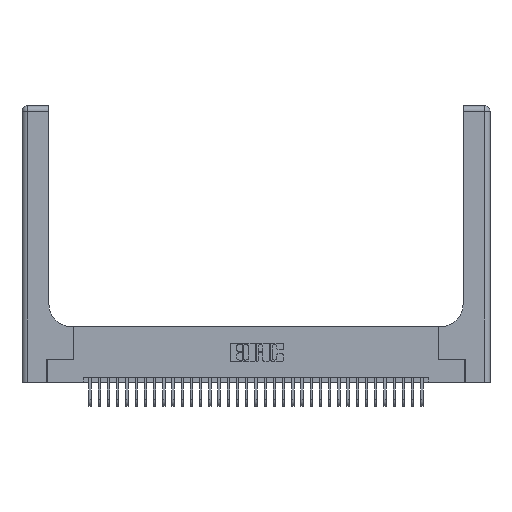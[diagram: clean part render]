
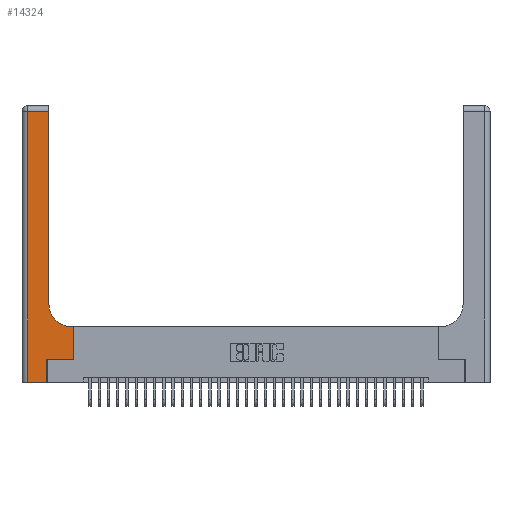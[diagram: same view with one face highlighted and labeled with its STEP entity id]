
A CAD part, top view. The second image highlights one B-rep face of the part: STEP entity #14324.
In plain terms, the highlighted planar face has unit normal (0, 0, 1).
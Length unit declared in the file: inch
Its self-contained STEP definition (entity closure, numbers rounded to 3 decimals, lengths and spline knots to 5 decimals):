
#932 = DIRECTION ( 'NONE',  ( 1., 0., 0. ) ) ;
#1067 = ORIENTED_EDGE ( 'NONE', *, *, #11201, .T. ) ;
#1811 = VECTOR ( 'NONE', #33774, 39.37008 ) ;
#1850 = CARTESIAN_POINT ( 'NONE',  ( 0., 0., 0.37 ) ) ;
#2205 = EDGE_CURVE ( 'NONE', #10153, #10173, #7530, .T. ) ;
#2216 = VECTOR ( 'NONE', #6789, 39.37008 ) ;
#2232 = ORIENTED_EDGE ( 'NONE', *, *, #28608, .T. ) ;
#2854 = VECTOR ( 'NONE', #29678, 39.37008 ) ;
#2979 = AXIS2_PLACEMENT_3D ( 'NONE', #20899, #5239, #23478 ) ;
#3751 = VECTOR ( 'NONE', #20194, 39.37008 ) ;
#5239 = DIRECTION ( 'NONE',  ( 0., 0., -1. ) ) ;
#5244 = EDGE_LOOP ( 'NONE', ( #20873, #32970, #9070, #2232, #15638, #33032, #24427, #32027, #1067 ) ) ;
#6436 = VERTEX_POINT ( 'NONE', #19688 ) ;
#6688 = CARTESIAN_POINT ( 'NONE',  ( 0.5585, 0.25, 0.37 ) ) ;
#6713 = EDGE_CURVE ( 'NONE', #10173, #20975, #14974, .T. ) ;
#6789 = DIRECTION ( 'NONE',  ( 0., 1., 0. ) ) ;
#6924 = DIRECTION ( 'NONE',  ( -1., 0., 0. ) ) ;
#6925 = EDGE_CURVE ( 'NONE', #18355, #10153, #29139, .T. ) ;
#7143 = CARTESIAN_POINT ( 'NONE',  ( 0.269, 0., 0.37 ) ) ;
#7530 = LINE ( 'NONE', #20809, #27480 ) ;
#7787 = CARTESIAN_POINT ( 'NONE',  ( 0.5585, 0.6, 0.37 ) ) ;
#8911 = CARTESIAN_POINT ( 'NONE',  ( 0.2915, 3., 0.37 ) ) ;
#8939 = CARTESIAN_POINT ( 'NONE',  ( 0.2915, 0.6, 0.37 ) ) ;
#9070 = ORIENTED_EDGE ( 'NONE', *, *, #31982, .T. ) ;
#9099 = LINE ( 'NONE', #1850, #3751 ) ;
#9261 = EDGE_CURVE ( 'NONE', #20975, #27877, #24466, .T. ) ;
#9428 = FACE_OUTER_BOUND ( 'NONE', #5244, .T. ) ;
#10153 = VERTEX_POINT ( 'NONE', #22305 ) ;
#10173 = VERTEX_POINT ( 'NONE', #6688 ) ;
#10424 = CARTESIAN_POINT ( 'NONE',  ( 0.269, 0., 0.37 ) ) ;
#10627 = VECTOR ( 'NONE', #11591, 39.37008 ) ;
#11201 = EDGE_CURVE ( 'NONE', #27877, #33024, #21081, .T. ) ;
#11591 = DIRECTION ( 'NONE',  ( -1., 0., 0. ) ) ;
#12222 = VERTEX_POINT ( 'NONE', #15811 ) ;
#13024 = PLANE ( 'NONE',  #2979 ) ;
#14324 = ADVANCED_FACE ( 'NONE', ( #9428 ), #13024, .F. ) ;
#14519 = CARTESIAN_POINT ( 'NONE',  ( 0.2915, 0.85, 0.37 ) ) ;
#14811 = AXIS2_PLACEMENT_3D ( 'NONE', #32173, #16679, #932 ) ;
#14974 = LINE ( 'NONE', #18310, #1811 ) ;
#15638 = ORIENTED_EDGE ( 'NONE', *, *, #6925, .T. ) ;
#15674 = EDGE_CURVE ( 'NONE', #12222, #18577, #30191, .T. ) ;
#15811 = CARTESIAN_POINT ( 'NONE',  ( 0.2915, 2.94, 0.37 ) ) ;
#15838 = CARTESIAN_POINT ( 'NONE',  ( 0.06, 3., 0.37 ) ) ;
#16679 = DIRECTION ( 'NONE',  ( 0., 0., -1. ) ) ;
#18310 = CARTESIAN_POINT ( 'NONE',  ( 0.5585, 0.25, 0.37 ) ) ;
#18355 = VERTEX_POINT ( 'NONE', #7143 ) ;
#18451 = LINE ( 'NONE', #8911, #2854 ) ;
#18577 = VERTEX_POINT ( 'NONE', #23644 ) ;
#19688 = CARTESIAN_POINT ( 'NONE',  ( 0.06, 0., 0.37 ) ) ;
#19792 = CARTESIAN_POINT ( 'NONE',  ( 0.5415, 0.6, 0.37 ) ) ;
#20194 = DIRECTION ( 'NONE',  ( 1., 0., 0. ) ) ;
#20809 = CARTESIAN_POINT ( 'NONE',  ( 0.269, 0.25, 0.37 ) ) ;
#20873 = ORIENTED_EDGE ( 'NONE', *, *, #23647, .T. ) ;
#20899 = CARTESIAN_POINT ( 'NONE',  ( 0., 3., 0.37 ) ) ;
#20975 = VERTEX_POINT ( 'NONE', #7787 ) ;
#21081 = CIRCLE ( 'NONE', #14811, 0.25 ) ;
#22305 = CARTESIAN_POINT ( 'NONE',  ( 0.269, 0.25, 0.37 ) ) ;
#22549 = CARTESIAN_POINT ( 'NONE',  ( 0., 2.94, 0.37 ) ) ;
#23288 = DIRECTION ( 'NONE',  ( 1., 0., 0. ) ) ;
#23478 = DIRECTION ( 'NONE',  ( -1., 0., 0. ) ) ;
#23644 = CARTESIAN_POINT ( 'NONE',  ( 0.06, 2.94, 0.37 ) ) ;
#23647 = EDGE_CURVE ( 'NONE', #33024, #12222, #18451, .T. ) ;
#23944 = VECTOR ( 'NONE', #31557, 39.37008 ) ;
#24170 = VECTOR ( 'NONE', #6924, 39.37008 ) ;
#24427 = ORIENTED_EDGE ( 'NONE', *, *, #6713, .T. ) ;
#24466 = LINE ( 'NONE', #8939, #10627 ) ;
#27480 = VECTOR ( 'NONE', #23288, 39.37008 ) ;
#27877 = VERTEX_POINT ( 'NONE', #19792 ) ;
#28608 = EDGE_CURVE ( 'NONE', #6436, #18355, #9099, .T. ) ;
#29139 = LINE ( 'NONE', #10424, #2216 ) ;
#29177 = LINE ( 'NONE', #15838, #23944 ) ;
#29678 = DIRECTION ( 'NONE',  ( 0., 1., 0. ) ) ;
#30191 = LINE ( 'NONE', #22549, #24170 ) ;
#31557 = DIRECTION ( 'NONE',  ( 0., -1., 0. ) ) ;
#31982 = EDGE_CURVE ( 'NONE', #18577, #6436, #29177, .T. ) ;
#32027 = ORIENTED_EDGE ( 'NONE', *, *, #9261, .T. ) ;
#32173 = CARTESIAN_POINT ( 'NONE',  ( 0.5415, 0.85, 0.37 ) ) ;
#32970 = ORIENTED_EDGE ( 'NONE', *, *, #15674, .T. ) ;
#33024 = VERTEX_POINT ( 'NONE', #14519 ) ;
#33032 = ORIENTED_EDGE ( 'NONE', *, *, #2205, .T. ) ;
#33774 = DIRECTION ( 'NONE',  ( 0., 1., 0. ) ) ;
